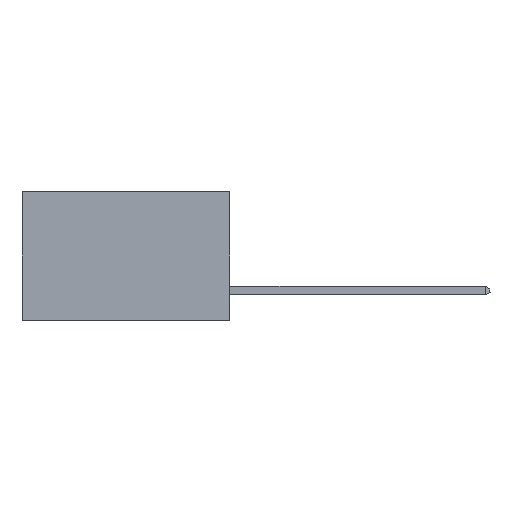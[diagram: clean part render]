
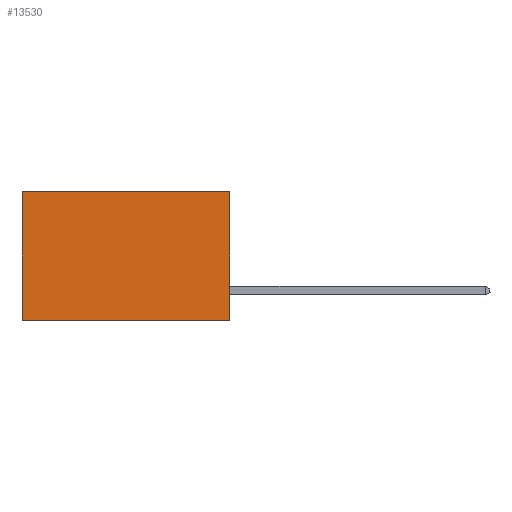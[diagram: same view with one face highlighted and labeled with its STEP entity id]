
A CAD part, left-side view. The second image highlights one B-rep face of the part: STEP entity #13530.
In plain terms, the highlighted planar face has unit normal (-1, 0, 0).
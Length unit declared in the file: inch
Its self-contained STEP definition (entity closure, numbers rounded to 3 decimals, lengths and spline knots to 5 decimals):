
#273 = VECTOR ( 'NONE', #13731, 39.37008 ) ;
#481 = VECTOR ( 'NONE', #6963, 39.37008 ) ;
#499 = ORIENTED_EDGE ( 'NONE', *, *, #14177, .F. ) ;
#725 = EDGE_CURVE ( 'NONE', #13568, #2028, #8960, .T. ) ;
#850 = AXIS2_PLACEMENT_3D ( 'NONE', #1466, #14555, #14604 ) ;
#882 = CARTESIAN_POINT ( 'NONE',  ( 0.298, 0.6, -0.37 ) ) ;
#1264 = FACE_OUTER_BOUND ( 'NONE', #11051, .T. ) ;
#1466 = CARTESIAN_POINT ( 'NONE',  ( 0.298, 0., 0. ) ) ;
#1934 = VERTEX_POINT ( 'NONE', #882 ) ;
#1942 = LINE ( 'NONE', #2652, #14204 ) ;
#2028 = VERTEX_POINT ( 'NONE', #2195 ) ;
#2195 = CARTESIAN_POINT ( 'NONE',  ( 0.298, 0.6, 0. ) ) ;
#2537 = LINE ( 'NONE', #11226, #273 ) ;
#2652 = CARTESIAN_POINT ( 'NONE',  ( 0.298, 0., -0.37 ) ) ;
#2716 = VERTEX_POINT ( 'NONE', #8390 ) ;
#3189 = CARTESIAN_POINT ( 'NONE',  ( 0.298, 0., 0. ) ) ;
#5131 = EDGE_CURVE ( 'NONE', #2716, #1934, #1942, .T. ) ;
#5633 = ORIENTED_EDGE ( 'NONE', *, *, #14737, .T. ) ;
#5734 = CARTESIAN_POINT ( 'NONE',  ( 0.298, 0., 0. ) ) ;
#6136 = ORIENTED_EDGE ( 'NONE', *, *, #5131, .F. ) ;
#6183 = ORIENTED_EDGE ( 'NONE', *, *, #725, .T. ) ;
#6748 = DIRECTION ( 'NONE',  ( 0., 1., 0. ) ) ;
#6963 = DIRECTION ( 'NONE',  ( 0., 0., -1. ) ) ;
#7421 = PLANE ( 'NONE',  #850 ) ;
#8390 = CARTESIAN_POINT ( 'NONE',  ( 0.298, 0., -0.37 ) ) ;
#8606 = VECTOR ( 'NONE', #6748, 39.37008 ) ;
#8960 = LINE ( 'NONE', #3189, #8606 ) ;
#9072 = CARTESIAN_POINT ( 'NONE',  ( 0.298, 0., 0. ) ) ;
#11051 = EDGE_LOOP ( 'NONE', ( #5633, #6136, #499, #6183 ) ) ;
#11109 = DIRECTION ( 'NONE',  ( 0., 1., 0. ) ) ;
#11226 = CARTESIAN_POINT ( 'NONE',  ( 0.298, 0.6, 0. ) ) ;
#12215 = LINE ( 'NONE', #5734, #481 ) ;
#13530 = ADVANCED_FACE ( 'NONE', ( #1264 ), #7421, .F. ) ;
#13568 = VERTEX_POINT ( 'NONE', #9072 ) ;
#13731 = DIRECTION ( 'NONE',  ( 0., 0., -1. ) ) ;
#14177 = EDGE_CURVE ( 'NONE', #13568, #2716, #12215, .T. ) ;
#14204 = VECTOR ( 'NONE', #11109, 39.37008 ) ;
#14555 = DIRECTION ( 'NONE',  ( 1., 0., 0. ) ) ;
#14604 = DIRECTION ( 'NONE',  ( 0., 0., -1. ) ) ;
#14737 = EDGE_CURVE ( 'NONE', #2028, #1934, #2537, .T. ) ;
